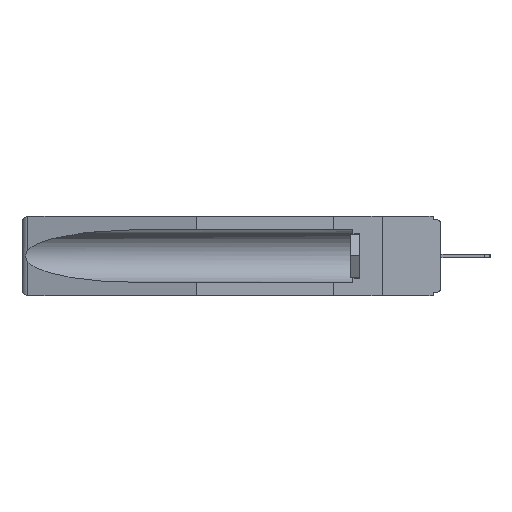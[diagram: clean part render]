
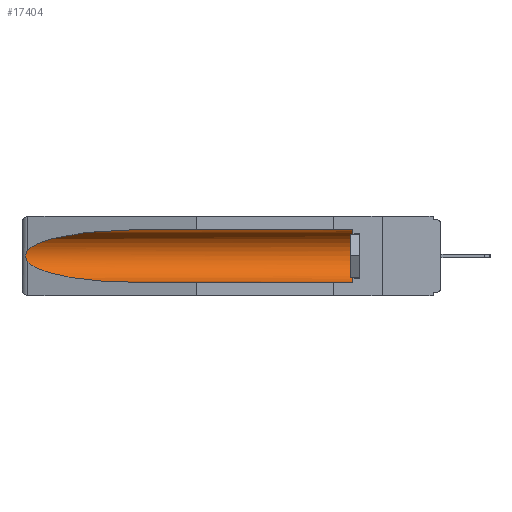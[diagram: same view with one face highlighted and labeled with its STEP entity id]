
A CAD part, left-side view. The second image highlights one B-rep face of the part: STEP entity #17404.
In plain terms, the highlighted cylindrical face has radius 2.857 mm (diameter 5.715 mm), a partial arc.
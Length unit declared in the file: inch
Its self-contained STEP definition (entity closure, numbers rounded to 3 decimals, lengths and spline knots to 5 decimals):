
#608 = CARTESIAN_POINT ( 'NONE',  ( 0.26537, 1.52718, -0.19328 ) ) ;
#624 = CARTESIAN_POINT ( 'NONE',  ( 0.155, -0.30754, -0.1715 ) ) ;
#853 = LINE ( 'NONE', #14080, #13451 ) ;
#1525 = CARTESIAN_POINT ( 'NONE',  ( 0.155, 0.126, -0.1715 ) ) ;
#2012 = CARTESIAN_POINT ( 'NONE',  ( 0.26597, 1.5296, -0.19026 ) ) ;
#2103 = VERTEX_POINT ( 'NONE', #9034 ) ;
#2153 = CARTESIAN_POINT ( 'NONE',  ( 0.26537, 1.52718, -0.14972 ) ) ;
#2962 = CARTESIAN_POINT ( 'NONE',  ( 0.2673, 1.5327, -0.16383 ) ) ;
#3793 = EDGE_LOOP ( 'NONE', ( #15407, #13739, #22264, #24539, #19743, #20223 ) ) ;
#3859 = DIRECTION ( 'NONE',  ( 0., -1., 0. ) ) ;
#4062 = EDGE_CURVE ( 'NONE', #14462, #27268, #25555, .T. ) ;
#4417 = CARTESIAN_POINT ( 'NONE',  ( 0.25451, 1.48313, -0.24835 ) ) ;
#5519 = CARTESIAN_POINT ( 'NONE',  ( 0.155, 0.126, -0.284 ) ) ;
#6627 =( BOUNDED_CURVE ( )  B_SPLINE_CURVE ( 3, ( #7336, #22564, #20527, #27242 ),
 .UNSPECIFIED., .F., .T. ) 
 B_SPLINE_CURVE_WITH_KNOTS ( ( 4, 4 ),
 ( 4.71239, 6.08839 ),
 .UNSPECIFIED. ) 
 CURVE ( )  GEOMETRIC_REPRESENTATION_ITEM ( )  RATIONAL_B_SPLINE_CURVE ( ( 1., 0.848, 0.848, 1. ) ) 
 REPRESENTATION_ITEM ( '' )  );
#7336 = CARTESIAN_POINT ( 'NONE',  ( 0.155, 1.07973, -0.059 ) ) ;
#7996 = B_SPLINE_CURVE_WITH_KNOTS ( 'NONE', 3,
 ( #2153, #24921, #22872, #2962, #11815, #20666, #25202, #21900, #2012, #8692 ),
 .UNSPECIFIED., .F., .F.,
 ( 4, 2, 2, 2, 4 ),
 ( 0., 0.00029, 0.00058, 0.00087, 0.00117 ),
 .UNSPECIFIED. ) ;
#8079 = CARTESIAN_POINT ( 'NONE',  ( 0.155, 1.07973, -0.284 ) ) ;
#8178 = EDGE_CURVE ( 'NONE', #21459, #8401, #25776, .T. ) ;
#8401 = VERTEX_POINT ( 'NONE', #18473 ) ;
#8692 = CARTESIAN_POINT ( 'NONE',  ( 0.26537, 1.52718, -0.19328 ) ) ;
#9034 = CARTESIAN_POINT ( 'NONE',  ( 0.155, 1.07973, -0.059 ) ) ;
#9191 = VERTEX_POINT ( 'NONE', #17053 ) ;
#9476 = DIRECTION ( 'NONE',  ( 0., 0., 1. ) ) ;
#9755 = VECTOR ( 'NONE', #27825, 39.37008 ) ;
#11815 = CARTESIAN_POINT ( 'NONE',  ( 0.2675, 1.53308, -0.16763 ) ) ;
#12854 = DIRECTION ( 'NONE',  ( 0., 0., 1. ) ) ;
#13233 = AXIS2_PLACEMENT_3D ( 'NONE', #1525, #3859, #12854 ) ;
#13451 = VECTOR ( 'NONE', #19008, 39.37008 ) ;
#13739 = ORIENTED_EDGE ( 'NONE', *, *, #21814, .T. ) ;
#13926 = AXIS2_PLACEMENT_3D ( 'NONE', #624, #28058, #9476 ) ;
#14080 = CARTESIAN_POINT ( 'NONE',  ( 0.155, -0.30754, -0.059 ) ) ;
#14462 = VERTEX_POINT ( 'NONE', #20241 ) ;
#15407 = ORIENTED_EDGE ( 'NONE', *, *, #19679, .T. ) ;
#17053 = CARTESIAN_POINT ( 'NONE',  ( 0.26537, 1.52718, -0.14972 ) ) ;
#17404 = ADVANCED_FACE ( 'NONE', ( #20512 ), #28201, .F. ) ;
#18473 = CARTESIAN_POINT ( 'NONE',  ( 0.155, 0.126, -0.059 ) ) ;
#18938 = CARTESIAN_POINT ( 'NONE',  ( 0.155, -0.30754, -0.284 ) ) ;
#19008 = DIRECTION ( 'NONE',  ( 0., 1., 0. ) ) ;
#19679 = EDGE_CURVE ( 'NONE', #2103, #9191, #6627, .T. ) ;
#19743 = ORIENTED_EDGE ( 'NONE', *, *, #8178, .T. ) ;
#20081 = CARTESIAN_POINT ( 'NONE',  ( 0.21114, 1.30732, -0.284 ) ) ;
#20223 = ORIENTED_EDGE ( 'NONE', *, *, #22651, .T. ) ;
#20241 = CARTESIAN_POINT ( 'NONE',  ( 0.26537, 1.52718, -0.19328 ) ) ;
#20512 = FACE_OUTER_BOUND ( 'NONE', #3793, .T. ) ;
#20527 = CARTESIAN_POINT ( 'NONE',  ( 0.25451, 1.48313, -0.09465 ) ) ;
#20666 = CARTESIAN_POINT ( 'NONE',  ( 0.2675, 1.53308, -0.17534 ) ) ;
#21111 = LINE ( 'NONE', #18938, #9755 ) ;
#21459 = VERTEX_POINT ( 'NONE', #5519 ) ;
#21814 = EDGE_CURVE ( 'NONE', #9191, #14462, #7996, .T. ) ;
#21900 = CARTESIAN_POINT ( 'NONE',  ( 0.26655, 1.53094, -0.18657 ) ) ;
#22264 = ORIENTED_EDGE ( 'NONE', *, *, #4062, .T. ) ;
#22564 = CARTESIAN_POINT ( 'NONE',  ( 0.21114, 1.30732, -0.059 ) ) ;
#22651 = EDGE_CURVE ( 'NONE', #8401, #2103, #853, .T. ) ;
#22872 = CARTESIAN_POINT ( 'NONE',  ( 0.26654, 1.53092, -0.15636 ) ) ;
#23760 = EDGE_CURVE ( 'NONE', #21459, #27268, #21111, .T. ) ;
#24539 = ORIENTED_EDGE ( 'NONE', *, *, #23760, .F. ) ;
#24891 = CARTESIAN_POINT ( 'NONE',  ( 0.155, 1.07973, -0.284 ) ) ;
#24921 = CARTESIAN_POINT ( 'NONE',  ( 0.26597, 1.52961, -0.15275 ) ) ;
#25202 = CARTESIAN_POINT ( 'NONE',  ( 0.2673, 1.53269, -0.17917 ) ) ;
#25555 =( BOUNDED_CURVE ( )  B_SPLINE_CURVE ( 3, ( #608, #4417, #20081, #24891 ),
 .UNSPECIFIED., .F., .T. ) 
 B_SPLINE_CURVE_WITH_KNOTS ( ( 4, 4 ),
 ( 0.1948, 1.5708 ),
 .UNSPECIFIED. ) 
 CURVE ( )  GEOMETRIC_REPRESENTATION_ITEM ( )  RATIONAL_B_SPLINE_CURVE ( ( 1., 0.848, 0.848, 1. ) ) 
 REPRESENTATION_ITEM ( '' )  );
#25776 = CIRCLE ( 'NONE', #13233, 0.1125 ) ;
#27242 = CARTESIAN_POINT ( 'NONE',  ( 0.26537, 1.52718, -0.14972 ) ) ;
#27268 = VERTEX_POINT ( 'NONE', #8079 ) ;
#27825 = DIRECTION ( 'NONE',  ( 0., 1., 0. ) ) ;
#28058 = DIRECTION ( 'NONE',  ( 0., 1., 0. ) ) ;
#28201 = CYLINDRICAL_SURFACE ( 'NONE', #13926, 0.1125 ) ;
